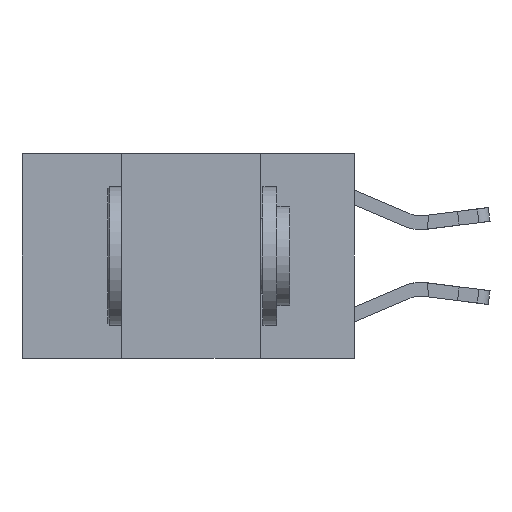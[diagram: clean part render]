
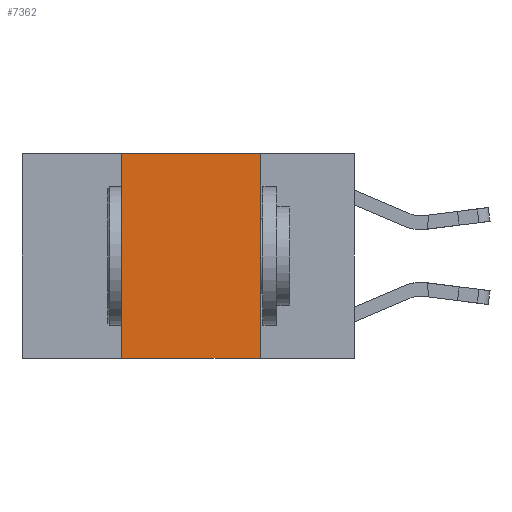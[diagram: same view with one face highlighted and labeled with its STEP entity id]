
A CAD part, left-side view. The second image highlights one B-rep face of the part: STEP entity #7362.
In plain terms, the highlighted planar face has unit normal (-1, 0, 0).
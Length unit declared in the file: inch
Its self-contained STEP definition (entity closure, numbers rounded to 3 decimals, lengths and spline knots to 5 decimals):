
#37 = PLANE ( 'NONE',  #5956 ) ;
#106 = EDGE_CURVE ( 'NONE', #12246, #13032, #11955, .T. ) ;
#440 = CARTESIAN_POINT ( 'NONE',  ( 0., 0.6, 0. ) ) ;
#1678 = EDGE_CURVE ( 'NONE', #13062, #7022, #8138, .T. ) ;
#1795 = ORIENTED_EDGE ( 'NONE', *, *, #11597, .F. ) ;
#1810 = ORIENTED_EDGE ( 'NONE', *, *, #10923, .F. ) ;
#3036 = LINE ( 'NONE', #8816, #4527 ) ;
#3108 = DIRECTION ( 'NONE',  ( 0., 0., -1. ) ) ;
#3569 = CARTESIAN_POINT ( 'NONE',  ( 0., 0.42, -0.37 ) ) ;
#4527 = VECTOR ( 'NONE', #3108, 39.37008 ) ;
#4612 = DIRECTION ( 'NONE',  ( 0., 0., 1. ) ) ;
#5070 = DIRECTION ( 'NONE',  ( 0., -1., 0. ) ) ;
#5356 = ORIENTED_EDGE ( 'NONE', *, *, #106, .F. ) ;
#5956 = AXIS2_PLACEMENT_3D ( 'NONE', #10286, #8979, #14752 ) ;
#7022 = VERTEX_POINT ( 'NONE', #11579 ) ;
#7312 = LINE ( 'NONE', #13943, #13871 ) ;
#7362 = ADVANCED_FACE ( 'NONE', ( #9127 ), #37, .F. ) ;
#7845 = VECTOR ( 'NONE', #5070, 39.37008 ) ;
#8138 = LINE ( 'NONE', #14147, #8207 ) ;
#8207 = VECTOR ( 'NONE', #8362, 39.37008 ) ;
#8362 = DIRECTION ( 'NONE',  ( 0., -1., 0. ) ) ;
#8816 = CARTESIAN_POINT ( 'NONE',  ( 0., 0.17, 0. ) ) ;
#8979 = DIRECTION ( 'NONE',  ( 1., 0., 0. ) ) ;
#9086 = EDGE_LOOP ( 'NONE', ( #1795, #5356, #1810, #12160 ) ) ;
#9127 = FACE_OUTER_BOUND ( 'NONE', #9086, .T. ) ;
#10286 = CARTESIAN_POINT ( 'NONE',  ( 0., 0.6, 0. ) ) ;
#10923 = EDGE_CURVE ( 'NONE', #13062, #12246, #7312, .T. ) ;
#11579 = CARTESIAN_POINT ( 'NONE',  ( 0., 0.17, -0.37 ) ) ;
#11597 = EDGE_CURVE ( 'NONE', #13032, #7022, #3036, .T. ) ;
#11955 = LINE ( 'NONE', #440, #7845 ) ;
#12160 = ORIENTED_EDGE ( 'NONE', *, *, #1678, .T. ) ;
#12246 = VERTEX_POINT ( 'NONE', #12587 ) ;
#12587 = CARTESIAN_POINT ( 'NONE',  ( 0., 0.42, 0. ) ) ;
#13032 = VERTEX_POINT ( 'NONE', #13829 ) ;
#13062 = VERTEX_POINT ( 'NONE', #3569 ) ;
#13829 = CARTESIAN_POINT ( 'NONE',  ( 0., 0.17, 0. ) ) ;
#13871 = VECTOR ( 'NONE', #4612, 39.37008 ) ;
#13943 = CARTESIAN_POINT ( 'NONE',  ( 0., 0.42, 0. ) ) ;
#14147 = CARTESIAN_POINT ( 'NONE',  ( 0., 0.6, -0.37 ) ) ;
#14752 = DIRECTION ( 'NONE',  ( 0., 0., -1. ) ) ;
